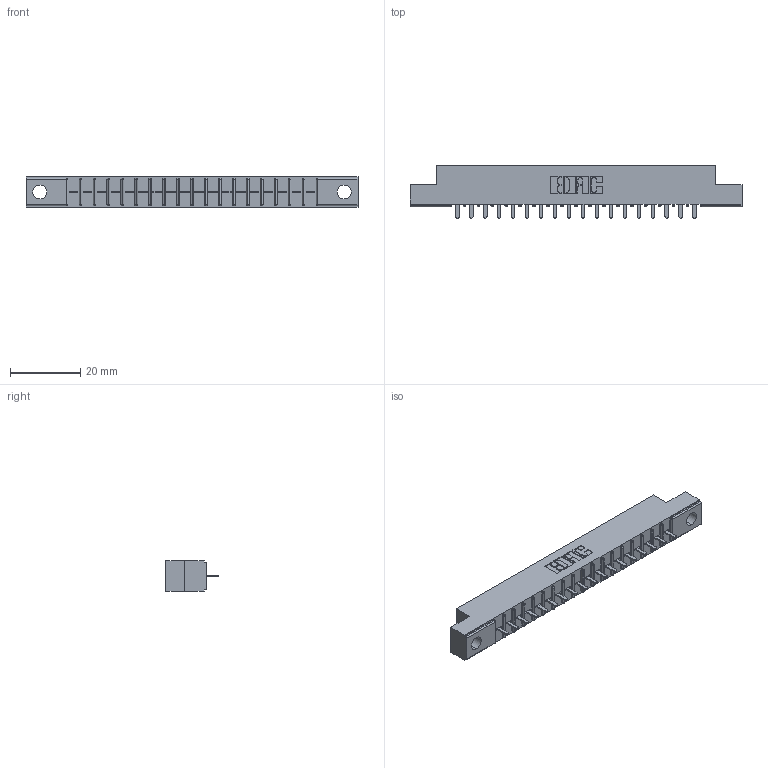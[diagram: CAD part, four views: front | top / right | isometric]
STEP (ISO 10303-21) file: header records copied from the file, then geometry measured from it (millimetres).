
FILE_DESCRIPTION (( 'STEP AP203' ), '1' );
FILE_NAME ('356-018-421-104.STEP', '2020-09-23T13:38:31', ( '' ), ( '' ), 'SwSTEP 2.0', 'SolidWorks 2020', '' );
FILE_SCHEMA (( 'CONFIG_CONTROL_DESIGN' ));
Length unit declared in the file: inch
Products named in the file (3): 306-290-001_121; 306 Part_.156 Dia; 356-018-421-104
Assembly tree (19 placements, depth 2):
  356-018-421-104
    306 Part_.156 Dia
    306-290-001_121  x18
Bounding box: 94.34 x 14.88 x 8.71 mm (x, y, z)
Volume: 6301.1 mm3; surface area: 8937.3 mm2
Topology: 19 solids, 19 shells, 1390 faces, 3898 edges, 2500 vertices
Faces by surface type: plane 928, cylinder 390, sphere 72
Entity records: 20269 total; most frequent: CARTESIAN_POINT 3403, ORIENTED_EDGE 3368, DIRECTION 3350, EDGE_CURVE 1684, VECTOR 1312, LINE 1312, VERTEX_POINT 1072, AXIS2_PLACEMENT_3D 1019
